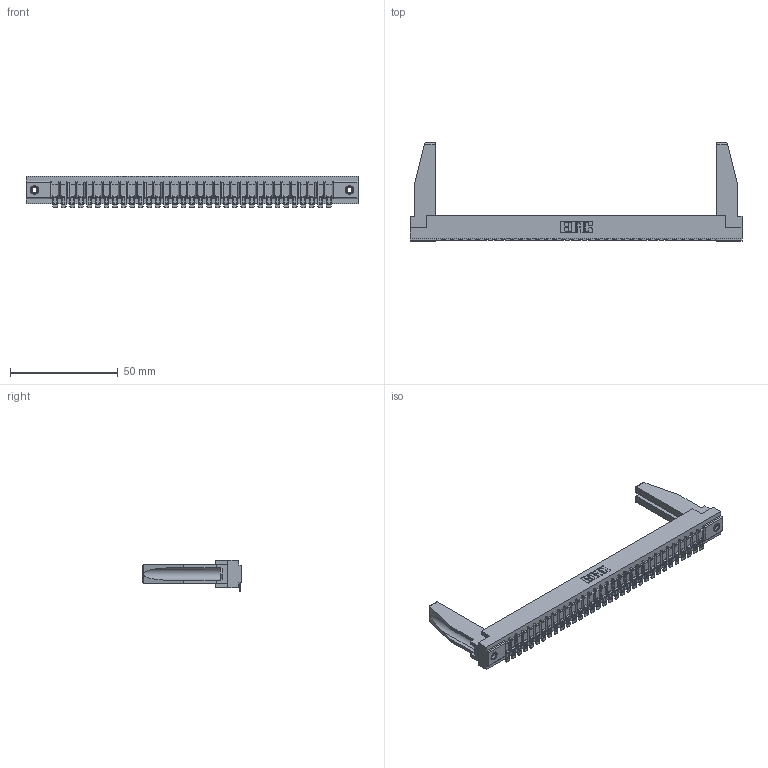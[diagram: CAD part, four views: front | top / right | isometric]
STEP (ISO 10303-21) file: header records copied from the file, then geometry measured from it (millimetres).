
FILE_DESCRIPTION (( 'STEP AP203' ), '1' );
FILE_NAME ('307-033-554-178.STEP', '2019-09-05T06:12:38', ( '' ), ( '' ), 'SwSTEP 2.0', 'SolidWorks 2016', '' );
FILE_SCHEMA (( 'CONFIG_CONTROL_DESIGN' ));
Length unit declared in the file: inch
Products named in the file (5): 307-220-078; 307-290-002_554; 307 Part_.156 Dia Mounting Holes; 345-250-001_345-250-001-102; 307-033-554-178
Assembly tree (38 placements, depth 2):
  307-033-554-178
    307 Part_.156 Dia Mounting Holes
    307-290-002_554  x33
    307-220-078  x2
    345-250-001_345-250-001-102  x2
Bounding box: 153.77 x 45.72 x 14.52 mm (x, y, z)
Volume: 20393.6 mm3; surface area: 24376.4 mm2
Topology: 38 solids, 38 shells, 2955 faces, 9002 edges, 5900 vertices
Faces by surface type: plane 1672, cylinder 1199, sphere 68, cone 12, torus 4
Entity records: 32804 total; most frequent: CARTESIAN_POINT 5532, ORIENTED_EDGE 5478, DIRECTION 5341, EDGE_CURVE 2739, LINE 2091, VECTOR 2091, VERTEX_POINT 1774, AXIS2_PLACEMENT_3D 1625
